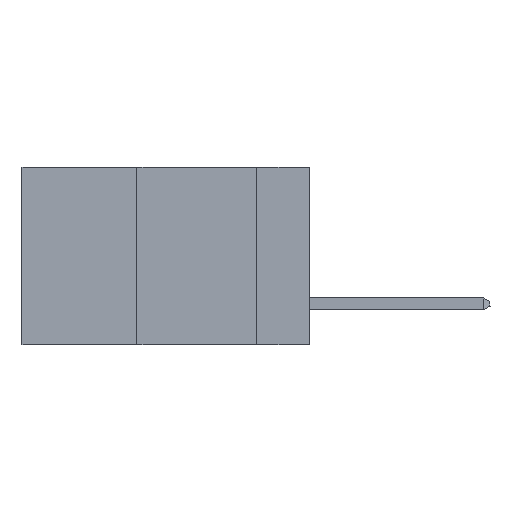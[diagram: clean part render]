
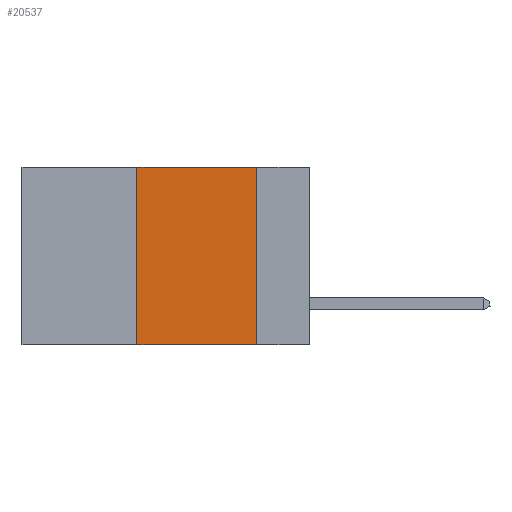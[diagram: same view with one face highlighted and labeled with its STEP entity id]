
A CAD part, left-side view. The second image highlights one B-rep face of the part: STEP entity #20537.
In plain terms, the highlighted planar face has unit normal (-1, 0, 0).
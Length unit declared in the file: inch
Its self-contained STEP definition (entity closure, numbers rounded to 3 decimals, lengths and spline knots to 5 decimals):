
#64 = CARTESIAN_POINT ( 'NONE',  ( 0., 0.6, -0.37 ) ) ;
#1661 = VERTEX_POINT ( 'NONE', #13786 ) ;
#2853 = LINE ( 'NONE', #17063, #20160 ) ;
#3005 = ORIENTED_EDGE ( 'NONE', *, *, #11721, .F. ) ;
#4676 = DIRECTION ( 'NONE',  ( 0., -1., 0. ) ) ;
#5097 = VERTEX_POINT ( 'NONE', #25666 ) ;
#5116 = ORIENTED_EDGE ( 'NONE', *, *, #9222, .F. ) ;
#5942 = DIRECTION ( 'NONE',  ( 0., -1., 0. ) ) ;
#6254 = FACE_OUTER_BOUND ( 'NONE', #21164, .T. ) ;
#7971 = EDGE_CURVE ( 'NONE', #23758, #24879, #2853, .T. ) ;
#8080 = DIRECTION ( 'NONE',  ( 0., 0., -1. ) ) ;
#8977 = AXIS2_PLACEMENT_3D ( 'NONE', #23760, #21581, #8080 ) ;
#9167 = CARTESIAN_POINT ( 'NONE',  ( 0., 0.36, 0. ) ) ;
#9222 = EDGE_CURVE ( 'NONE', #5097, #23758, #21756, .T. ) ;
#10280 = PLANE ( 'NONE',  #8977 ) ;
#10520 = VECTOR ( 'NONE', #24919, 39.37008 ) ;
#11721 = EDGE_CURVE ( 'NONE', #24879, #1661, #12464, .T. ) ;
#12464 = LINE ( 'NONE', #27063, #13168 ) ;
#13168 = VECTOR ( 'NONE', #20257, 39.37008 ) ;
#13478 = ORIENTED_EDGE ( 'NONE', *, *, #20909, .T. ) ;
#13786 = CARTESIAN_POINT ( 'NONE',  ( 0., 0.11, -0.37 ) ) ;
#14591 = VECTOR ( 'NONE', #4676, 39.37008 ) ;
#15276 = LINE ( 'NONE', #64, #14591 ) ;
#17063 = CARTESIAN_POINT ( 'NONE',  ( 0., 0.6, 0. ) ) ;
#20160 = VECTOR ( 'NONE', #5942, 39.37008 ) ;
#20257 = DIRECTION ( 'NONE',  ( 0., 0., -1. ) ) ;
#20456 = CARTESIAN_POINT ( 'NONE',  ( 0., 0.11, 0. ) ) ;
#20537 = ADVANCED_FACE ( 'NONE', ( #6254 ), #10280, .F. ) ;
#20909 = EDGE_CURVE ( 'NONE', #5097, #1661, #15276, .T. ) ;
#21164 = EDGE_LOOP ( 'NONE', ( #3005, #25236, #5116, #13478 ) ) ;
#21581 = DIRECTION ( 'NONE',  ( 1., 0., 0. ) ) ;
#21756 = LINE ( 'NONE', #9167, #10520 ) ;
#23061 = CARTESIAN_POINT ( 'NONE',  ( 0., 0.36, 0. ) ) ;
#23758 = VERTEX_POINT ( 'NONE', #23061 ) ;
#23760 = CARTESIAN_POINT ( 'NONE',  ( 0., 0.6, 0. ) ) ;
#24879 = VERTEX_POINT ( 'NONE', #20456 ) ;
#24919 = DIRECTION ( 'NONE',  ( 0., 0., 1. ) ) ;
#25236 = ORIENTED_EDGE ( 'NONE', *, *, #7971, .F. ) ;
#25666 = CARTESIAN_POINT ( 'NONE',  ( 0., 0.36, -0.37 ) ) ;
#27063 = CARTESIAN_POINT ( 'NONE',  ( 0., 0.11, 0. ) ) ;
